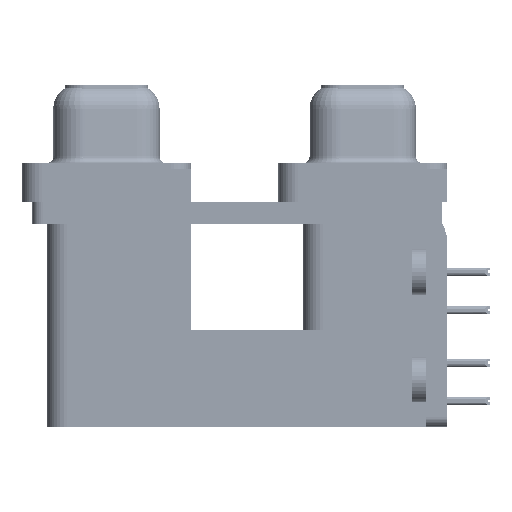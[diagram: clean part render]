
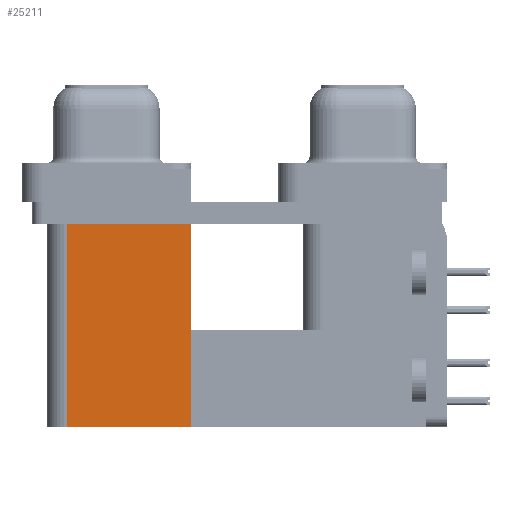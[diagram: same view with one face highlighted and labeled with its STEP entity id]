
A CAD part, left-side view. The second image highlights one B-rep face of the part: STEP entity #25211.
In plain terms, the highlighted planar face has unit normal (-1, 0, 0).
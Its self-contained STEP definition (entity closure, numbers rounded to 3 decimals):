
#333 = LINE ( 'NONE', #5502, #38227 ) ;
#2061 = CARTESIAN_POINT ( 'NONE',  ( 3.7, 12.775, -19.2 ) ) ;
#2812 = VECTOR ( 'NONE', #49979, 1000. ) ;
#3676 = VERTEX_POINT ( 'NONE', #36824 ) ;
#3730 = DIRECTION ( 'NONE',  ( 0., 0., 1. ) ) ;
#5502 = CARTESIAN_POINT ( 'NONE',  ( 3.7, 12.775, -19.2 ) ) ;
#7174 = VERTEX_POINT ( 'NONE', #8736 ) ;
#7927 = CARTESIAN_POINT ( 'NONE',  ( 3.7, 21.975, -2.5 ) ) ;
#8736 = CARTESIAN_POINT ( 'NONE',  ( 3.7, 12.775, -2.5 ) ) ;
#12226 = EDGE_CURVE ( 'NONE', #50029, #7174, #333, .T. ) ;
#12277 = CARTESIAN_POINT ( 'NONE',  ( 3.7, 12.775, -2.5 ) ) ;
#13082 = PLANE ( 'NONE',  #40310 ) ;
#13284 = CARTESIAN_POINT ( 'NONE',  ( 3.7, 12.775, -19.2 ) ) ;
#19915 = EDGE_CURVE ( 'NONE', #7174, #23127, #21444, .T. ) ;
#21444 = LINE ( 'NONE', #12277, #42935 ) ;
#22223 = FACE_OUTER_BOUND ( 'NONE', #60127, .T. ) ;
#23127 = VERTEX_POINT ( 'NONE', #7927 ) ;
#25211 = ADVANCED_FACE ( 'NONE', ( #22223 ), #13082, .F. ) ;
#26961 = CARTESIAN_POINT ( 'NONE',  ( 3.7, 21.975, -19.2 ) ) ;
#30057 = VECTOR ( 'NONE', #3730, 1000. ) ;
#31307 = LINE ( 'NONE', #13284, #2812 ) ;
#31694 = ORIENTED_EDGE ( 'NONE', *, *, #43523, .F. ) ;
#36824 = CARTESIAN_POINT ( 'NONE',  ( 3.7, 21.975, -19.2 ) ) ;
#38227 = VECTOR ( 'NONE', #51398, 1000. ) ;
#39044 = ORIENTED_EDGE ( 'NONE', *, *, #54921, .F. ) ;
#40310 = AXIS2_PLACEMENT_3D ( 'NONE', #58978, #50999, #50678 ) ;
#41745 = ORIENTED_EDGE ( 'NONE', *, *, #12226, .T. ) ;
#41944 = LINE ( 'NONE', #26961, #30057 ) ;
#42935 = VECTOR ( 'NONE', #44393, 1000. ) ;
#43523 = EDGE_CURVE ( 'NONE', #50029, #3676, #31307, .T. ) ;
#44393 = DIRECTION ( 'NONE',  ( 0., 1., 0. ) ) ;
#49979 = DIRECTION ( 'NONE',  ( 0., 1., 0. ) ) ;
#50029 = VERTEX_POINT ( 'NONE', #2061 ) ;
#50678 = DIRECTION ( 'NONE',  ( 0., 1., 0. ) ) ;
#50999 = DIRECTION ( 'NONE',  ( 1., 0., 0. ) ) ;
#51398 = DIRECTION ( 'NONE',  ( 0., 0., 1. ) ) ;
#53419 = ORIENTED_EDGE ( 'NONE', *, *, #19915, .T. ) ;
#54921 = EDGE_CURVE ( 'NONE', #3676, #23127, #41944, .T. ) ;
#58978 = CARTESIAN_POINT ( 'NONE',  ( 3.7, 12.775, -19.2 ) ) ;
#60127 = EDGE_LOOP ( 'NONE', ( #53419, #39044, #31694, #41745 ) ) ;
